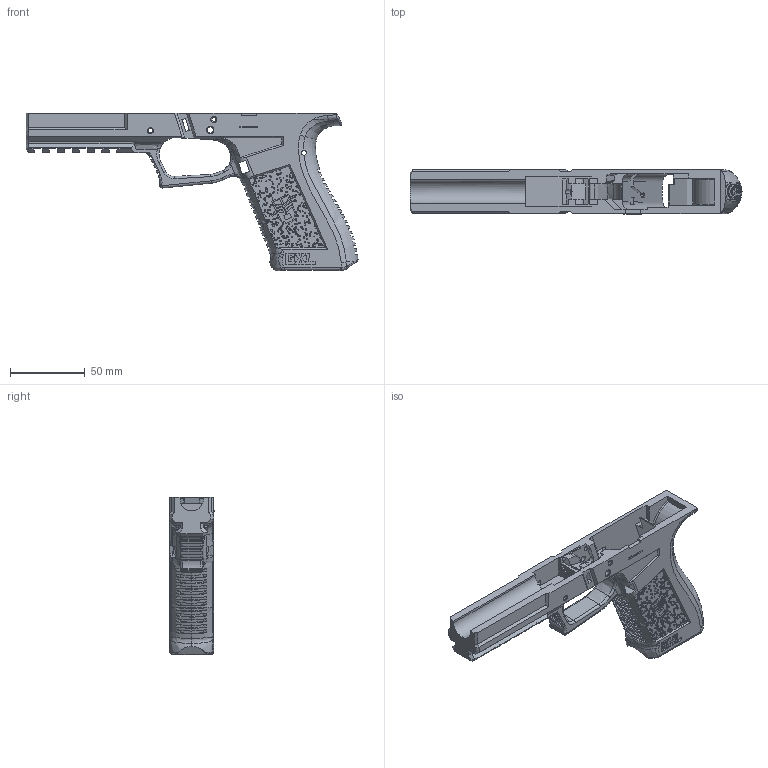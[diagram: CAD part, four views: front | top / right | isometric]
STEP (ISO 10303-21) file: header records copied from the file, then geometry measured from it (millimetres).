
FILE_DESCRIPTION(/* description */ (''),/* implementation_level */ '2;1');
FILE_NAME(/* name */ 'DD17.2 GXLR34.step',/* time_stamp */ '2022-07-31T09:39:56-05:00',/* author */ (''),/* organization */ (''),/* preprocessor_version */ 'ST-DEVELOPER v19',/* originating_system */ 'Autodesk Translation Framework v11.7.0.108',/* authorisation */ '');
FILE_SCHEMA (('AUTOMOTIVE_DESIGN { 1 0 10303 214 3 1 1 }'));
Products named in the file (1): DD17.2 SDI GXL/R
Bounding box: 221.76 x 29.73 x 104.95 mm (x, y, z)
Volume: 123913.4 mm3; surface area: 55977.5 mm2
Topology: 1 solids, 2 shells, 3421 faces, 8962 edges, 5923 vertices
Faces by surface type: bspline 2272, plane 1074, cylinder 64, torus 11
Full cylindrical faces by diameter (mm): 1.933 x1, 3 x4, 3.2 x2, 3.5 x1, 4.1 x2
Entity records: 137298 total; most frequent: CARTESIAN_POINT 75286, ORIENTED_EDGE 17906, EDGE_CURVE 8953, DIRECTION 6519, VERTEX_POINT 5923, EDGE_LOOP 3838, LINE 3725, VECTOR 3725
